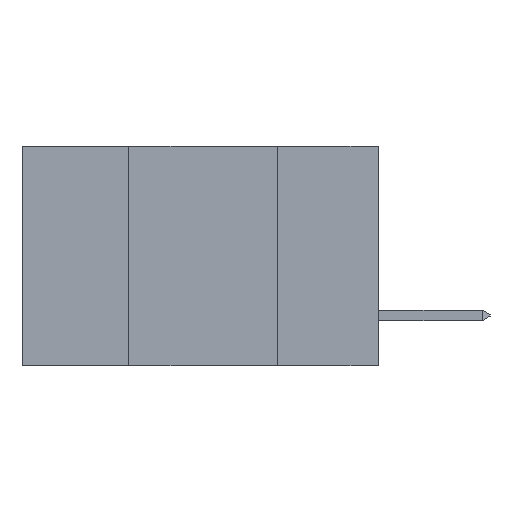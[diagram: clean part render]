
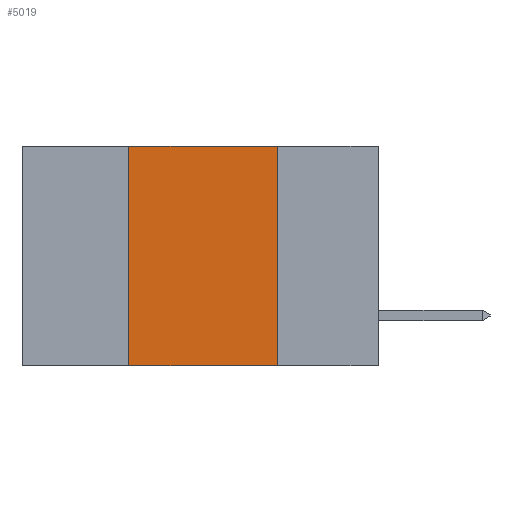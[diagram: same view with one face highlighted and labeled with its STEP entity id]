
A CAD part, left-side view. The second image highlights one B-rep face of the part: STEP entity #5019.
In plain terms, the highlighted planar face has unit normal (-1, 0, 0).
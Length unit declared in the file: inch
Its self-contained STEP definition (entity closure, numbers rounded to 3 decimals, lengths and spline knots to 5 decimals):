
#6 = EDGE_CURVE ( 'NONE', #13132, #7758, #7177, .T. ) ;
#264 = DIRECTION ( 'NONE',  ( 0., -1., 0. ) ) ;
#653 = PLANE ( 'NONE',  #4507 ) ;
#806 = EDGE_CURVE ( 'NONE', #13132, #6765, #824, .T. ) ;
#824 = LINE ( 'NONE', #2458, #1569 ) ;
#1228 = LINE ( 'NONE', #7005, #7515 ) ;
#1569 = VECTOR ( 'NONE', #2228, 39.37008 ) ;
#1605 = CARTESIAN_POINT ( 'NONE',  ( 0., 0.17, 0. ) ) ;
#1710 = CARTESIAN_POINT ( 'NONE',  ( 0., 0.6, -0.37 ) ) ;
#1983 = CARTESIAN_POINT ( 'NONE',  ( 0., 0.17, 0. ) ) ;
#2228 = DIRECTION ( 'NONE',  ( 0., 0., 1. ) ) ;
#2458 = CARTESIAN_POINT ( 'NONE',  ( 0., 0.42, 0. ) ) ;
#2689 = VECTOR ( 'NONE', #11917, 39.37008 ) ;
#3075 = EDGE_CURVE ( 'NONE', #12379, #7758, #11761, .T. ) ;
#3525 = ORIENTED_EDGE ( 'NONE', *, *, #6, .T. ) ;
#3611 = CARTESIAN_POINT ( 'NONE',  ( 0., 0.42, 0. ) ) ;
#4261 = DIRECTION ( 'NONE',  ( 0., -1., 0. ) ) ;
#4507 = AXIS2_PLACEMENT_3D ( 'NONE', #11224, #9843, #6043 ) ;
#5019 = ADVANCED_FACE ( 'NONE', ( #7625 ), #653, .F. ) ;
#5090 = EDGE_LOOP ( 'NONE', ( #10540, #5463, #5808, #3525 ) ) ;
#5463 = ORIENTED_EDGE ( 'NONE', *, *, #11361, .F. ) ;
#5808 = ORIENTED_EDGE ( 'NONE', *, *, #806, .F. ) ;
#6043 = DIRECTION ( 'NONE',  ( 0., 0., -1. ) ) ;
#6765 = VERTEX_POINT ( 'NONE', #3611 ) ;
#7005 = CARTESIAN_POINT ( 'NONE',  ( 0., 0.6, 0. ) ) ;
#7177 = LINE ( 'NONE', #1710, #12858 ) ;
#7515 = VECTOR ( 'NONE', #264, 39.37008 ) ;
#7625 = FACE_OUTER_BOUND ( 'NONE', #5090, .T. ) ;
#7758 = VERTEX_POINT ( 'NONE', #11292 ) ;
#8079 = CARTESIAN_POINT ( 'NONE',  ( 0., 0.42, -0.37 ) ) ;
#9843 = DIRECTION ( 'NONE',  ( 1., 0., 0. ) ) ;
#10540 = ORIENTED_EDGE ( 'NONE', *, *, #3075, .F. ) ;
#11224 = CARTESIAN_POINT ( 'NONE',  ( 0., 0.6, 0. ) ) ;
#11292 = CARTESIAN_POINT ( 'NONE',  ( 0., 0.17, -0.37 ) ) ;
#11361 = EDGE_CURVE ( 'NONE', #6765, #12379, #1228, .T. ) ;
#11761 = LINE ( 'NONE', #1605, #2689 ) ;
#11917 = DIRECTION ( 'NONE',  ( 0., 0., -1. ) ) ;
#12379 = VERTEX_POINT ( 'NONE', #1983 ) ;
#12858 = VECTOR ( 'NONE', #4261, 39.37008 ) ;
#13132 = VERTEX_POINT ( 'NONE', #8079 ) ;
